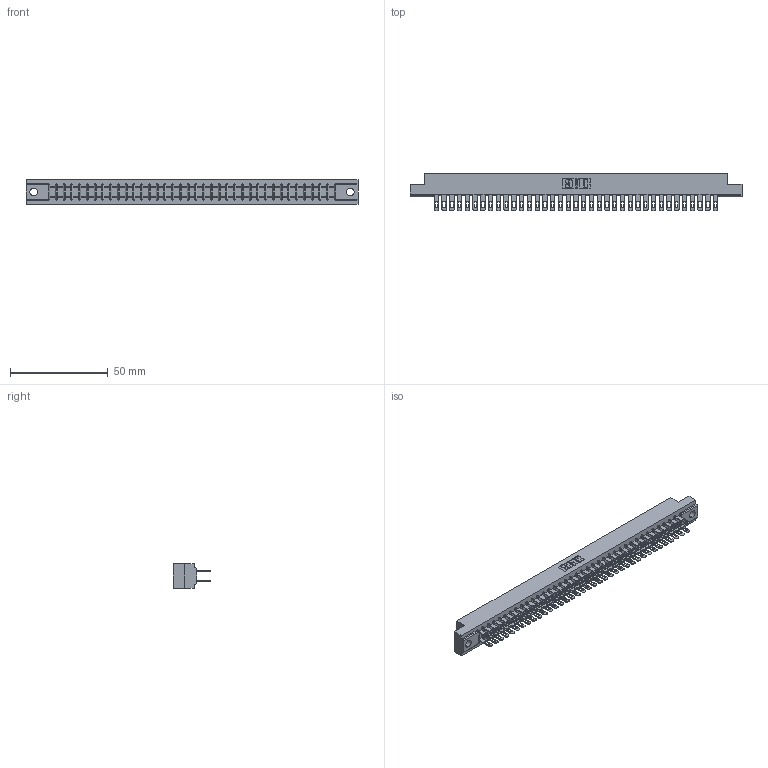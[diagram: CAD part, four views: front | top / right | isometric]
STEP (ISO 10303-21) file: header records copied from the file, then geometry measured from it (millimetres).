
FILE_DESCRIPTION (( 'STEP AP203' ), '1' );
FILE_NAME ('307-074-400-204.STEP', '2020-10-01T02:49:45', ( '' ), ( '' ), 'SwSTEP 2.0', 'SolidWorks 2020', '' );
FILE_SCHEMA (( 'CONFIG_CONTROL_DESIGN' ));
Length unit declared in the file: inch
Products named in the file (3): 307-074-400-204; 307-290-001_500; 307 Part_.156 Dia Mounting Holes
Assembly tree (75 placements, depth 2):
  307-074-400-204
    307 Part_.156 Dia Mounting Holes
    307-290-001_500  x74
Bounding box: 169.62 x 19.18 x 12.7 mm (x, y, z)
Volume: 18107.9 mm3; surface area: 23066.2 mm2
Topology: 75 solids, 75 shells, 3574 faces, 9979 edges, 6450 vertices
Faces by surface type: plane 2304, cylinder 1194, sphere 76
Entity records: 33912 total; most frequent: CARTESIAN_POINT 5551, ORIENTED_EDGE 5498, DIRECTION 5433, EDGE_CURVE 2749, LINE 2113, VECTOR 2113, VERTEX_POINT 1778, AXIS2_PLACEMENT_3D 1660
